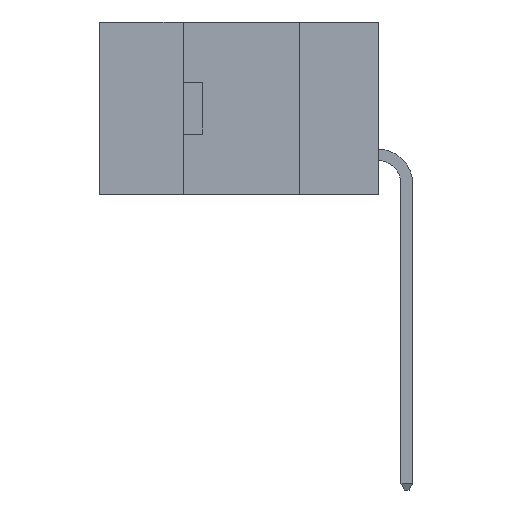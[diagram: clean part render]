
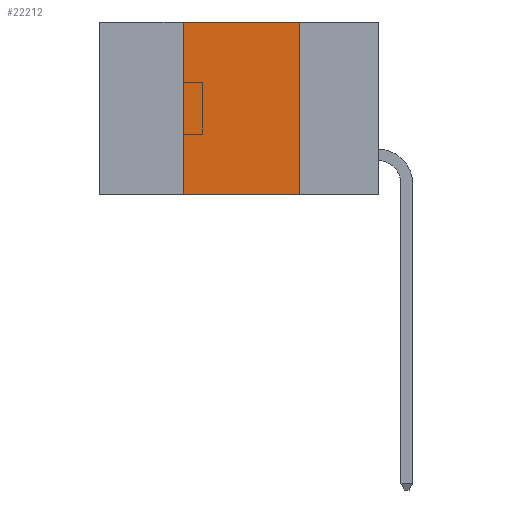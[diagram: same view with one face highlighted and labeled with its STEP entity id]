
A CAD part, left-side view. The second image highlights one B-rep face of the part: STEP entity #22212.
In plain terms, the highlighted planar face has unit normal (-1, 0, 0).
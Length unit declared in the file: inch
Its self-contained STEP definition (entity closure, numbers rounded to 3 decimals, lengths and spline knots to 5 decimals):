
#231 = EDGE_CURVE ( 'NONE', #658, #2947, #1087, .T. ) ;
#658 = VERTEX_POINT ( 'NONE', #4890 ) ;
#1087 = LINE ( 'NONE', #15709, #17332 ) ;
#1662 = DIRECTION ( 'NONE',  ( 0., 0., 1. ) ) ;
#2084 = DIRECTION ( 'NONE',  ( 1., 0., 0. ) ) ;
#2947 = VERTEX_POINT ( 'NONE', #20153 ) ;
#4116 = ORIENTED_EDGE ( 'NONE', *, *, #8393, .F. ) ;
#4884 = VECTOR ( 'NONE', #18898, 39.37008 ) ;
#4890 = CARTESIAN_POINT ( 'NONE',  ( 0., 0.42, -0.37 ) ) ;
#6614 = VECTOR ( 'NONE', #1662, 39.37008 ) ;
#7506 = CARTESIAN_POINT ( 'NONE',  ( 0., 0.42, 0. ) ) ;
#8023 = VECTOR ( 'NONE', #20813, 39.37008 ) ;
#8393 = EDGE_CURVE ( 'NONE', #18288, #16145, #10615, .T. ) ;
#10615 = LINE ( 'NONE', #22931, #4884 ) ;
#12110 = EDGE_LOOP ( 'NONE', ( #16711, #4116, #15158, #18309 ) ) ;
#12756 = PLANE ( 'NONE',  #22533 ) ;
#14214 = FACE_OUTER_BOUND ( 'NONE', #12110, .T. ) ;
#14419 = CARTESIAN_POINT ( 'NONE',  ( 0., 0.42, -0.37 ) ) ;
#14624 = CARTESIAN_POINT ( 'NONE',  ( 0., 0.17, -0.37 ) ) ;
#15158 = ORIENTED_EDGE ( 'NONE', *, *, #21410, .F. ) ;
#15709 = CARTESIAN_POINT ( 'NONE',  ( 0., 0.6, -0.37 ) ) ;
#16145 = VERTEX_POINT ( 'NONE', #19901 ) ;
#16313 = DIRECTION ( 'NONE',  ( 0., -1., 0. ) ) ;
#16711 = ORIENTED_EDGE ( 'NONE', *, *, #20906, .F. ) ;
#16899 = DIRECTION ( 'NONE',  ( 0., 0., -1. ) ) ;
#17145 = LINE ( 'NONE', #14419, #6614 ) ;
#17332 = VECTOR ( 'NONE', #16313, 39.37008 ) ;
#18288 = VERTEX_POINT ( 'NONE', #7506 ) ;
#18309 = ORIENTED_EDGE ( 'NONE', *, *, #231, .T. ) ;
#18898 = DIRECTION ( 'NONE',  ( 0., -1., 0. ) ) ;
#19724 = LINE ( 'NONE', #14624, #8023 ) ;
#19901 = CARTESIAN_POINT ( 'NONE',  ( 0., 0.17, 0. ) ) ;
#20153 = CARTESIAN_POINT ( 'NONE',  ( 0., 0.17, -0.37 ) ) ;
#20813 = DIRECTION ( 'NONE',  ( 0., 0., -1. ) ) ;
#20906 = EDGE_CURVE ( 'NONE', #16145, #2947, #19724, .T. ) ;
#21410 = EDGE_CURVE ( 'NONE', #658, #18288, #17145, .T. ) ;
#22212 = ADVANCED_FACE ( 'NONE', ( #14214 ), #12756, .F. ) ;
#22533 = AXIS2_PLACEMENT_3D ( 'NONE', #27054, #2084, #16899 ) ;
#22931 = CARTESIAN_POINT ( 'NONE',  ( 0., 0.6, 0. ) ) ;
#27054 = CARTESIAN_POINT ( 'NONE',  ( 0., 0.6, 0. ) ) ;
